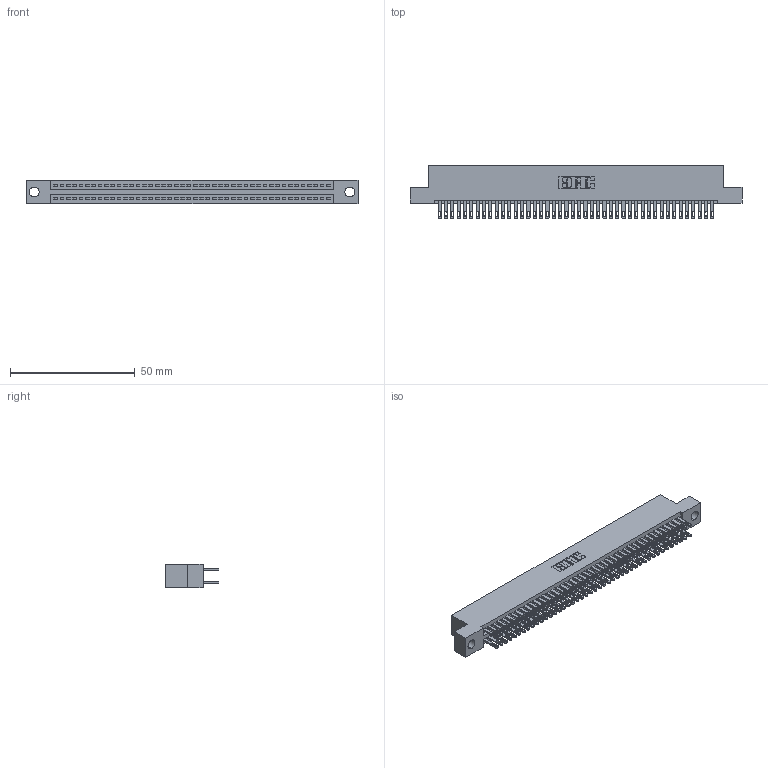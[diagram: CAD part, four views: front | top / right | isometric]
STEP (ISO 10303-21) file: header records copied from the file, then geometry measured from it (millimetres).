
FILE_DESCRIPTION (( 'STEP AP203' ), '1' );
FILE_NAME ('345-088-500-204.STEP', '2021-05-20T13:50:22', ( '' ), ( '' ), 'SwSTEP 2.0', 'SolidWorks 2020', '' );
FILE_SCHEMA (( 'CONFIG_CONTROL_DESIGN' ));
Length unit declared in the file: inch
Products named in the file (3): 345 Part_Flush Mounting Lugs - 0.156 Dia-TI; 345-088-500-204; 345-292-001_345-293-100
Assembly tree (89 placements, depth 2):
  345-088-500-204
    345 Part_Flush Mounting Lugs - 0.156 Dia-TI
    345-292-001_345-293-100  x88
Bounding box: 132.97 x 21.51 x 9.4 mm (x, y, z)
Volume: 13098.3 mm3; surface area: 20149.3 mm2
Topology: 89 solids, 89 shells, 4188 faces, 12785 edges, 8522 vertices
Faces by surface type: plane 2470, cylinder 1718
Entity records: 34603 total; most frequent: CARTESIAN_POINT 5802, ORIENTED_EDGE 5734, DIRECTION 5115, EDGE_CURVE 2867, VECTOR 2555, LINE 2555, VERTEX_POINT 1910, AXIS2_PLACEMENT_3D 1280
